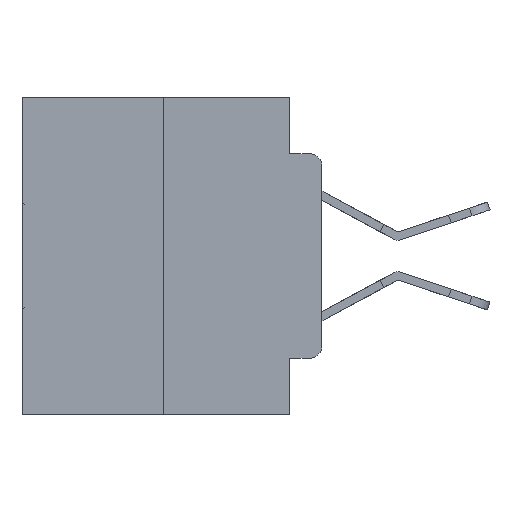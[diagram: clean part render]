
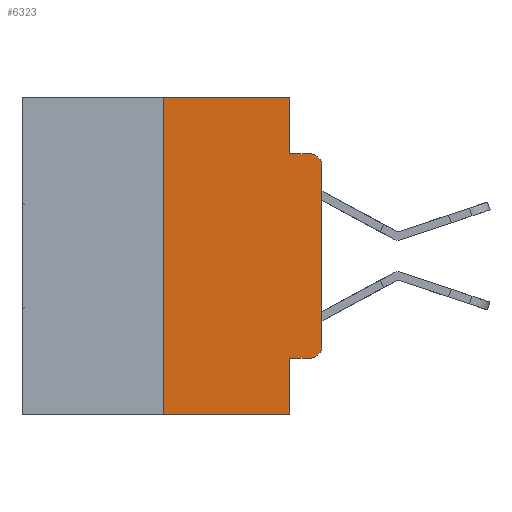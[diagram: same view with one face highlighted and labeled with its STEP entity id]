
A CAD part, left-side view. The second image highlights one B-rep face of the part: STEP entity #6323.
In plain terms, the highlighted planar face has unit normal (-1, 0, 0).
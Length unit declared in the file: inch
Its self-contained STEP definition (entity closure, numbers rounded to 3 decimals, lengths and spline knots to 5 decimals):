
#49 = CARTESIAN_POINT ( 'NONE',  ( 0., 0.02, -0.3915 ) ) ;
#117 = CARTESIAN_POINT ( 'NONE',  ( 0., 0., 0. ) ) ;
#957 = EDGE_CURVE ( 'NONE', #20070, #7459, #7566, .T. ) ;
#1238 = CARTESIAN_POINT ( 'NONE',  ( 0., 0., -0.3915 ) ) ;
#1252 = EDGE_LOOP ( 'NONE', ( #4710, #22778, #15737, #4703, #14623, #15390, #3046, #19075, #13625, #22520 ) ) ;
#1361 = CARTESIAN_POINT ( 'NONE',  ( 0., 0.051, -0.0885 ) ) ;
#1667 = VECTOR ( 'NONE', #22784, 39.37008 ) ;
#1804 = CARTESIAN_POINT ( 'NONE',  ( 0., 0.25, 0. ) ) ;
#1815 = CARTESIAN_POINT ( 'NONE',  ( 0., 0.02, -0.0885 ) ) ;
#1923 = AXIS2_PLACEMENT_3D ( 'NONE', #9170, #6244, #6087 ) ;
#2115 = VERTEX_POINT ( 'NONE', #1361 ) ;
#2383 = EDGE_CURVE ( 'NONE', #4412, #13299, #23079, .T. ) ;
#2407 = LINE ( 'NONE', #117, #4605 ) ;
#3046 = ORIENTED_EDGE ( 'NONE', *, *, #19888, .T. ) ;
#3507 = VECTOR ( 'NONE', #13472, 39.37008 ) ;
#4167 = DIRECTION ( 'NONE',  ( 0., 0., -1. ) ) ;
#4253 = PLANE ( 'NONE',  #1923 ) ;
#4412 = VERTEX_POINT ( 'NONE', #4802 ) ;
#4605 = VECTOR ( 'NONE', #20945, 39.37008 ) ;
#4703 = ORIENTED_EDGE ( 'NONE', *, *, #20330, .F. ) ;
#4710 = ORIENTED_EDGE ( 'NONE', *, *, #10643, .T. ) ;
#4802 = CARTESIAN_POINT ( 'NONE',  ( 0., 0.25, -0.5 ) ) ;
#5349 = CARTESIAN_POINT ( 'NONE',  ( 0., 0.02, -0.4115 ) ) ;
#6087 = DIRECTION ( 'NONE',  ( 0., 0., -1. ) ) ;
#6143 = DIRECTION ( 'NONE',  ( 0., -1., 0. ) ) ;
#6244 = DIRECTION ( 'NONE',  ( 1., 0., 0. ) ) ;
#6323 = ADVANCED_FACE ( 'NONE', ( #13639 ), #4253, .F. ) ;
#6870 = DIRECTION ( 'NONE',  ( 0., -1., 0. ) ) ;
#7145 = CARTESIAN_POINT ( 'NONE',  ( 0., 0.25, 0. ) ) ;
#7459 = VERTEX_POINT ( 'NONE', #5349 ) ;
#7566 = LINE ( 'NONE', #22283, #10491 ) ;
#7925 = CARTESIAN_POINT ( 'NONE',  ( 0., 0.051, -0.5 ) ) ;
#8088 = EDGE_CURVE ( 'NONE', #19661, #25781, #27586, .T. ) ;
#8768 = CARTESIAN_POINT ( 'NONE',  ( 0., 0.473, 0. ) ) ;
#9170 = CARTESIAN_POINT ( 'NONE',  ( 0., 0.473, 0. ) ) ;
#10226 = VECTOR ( 'NONE', #6143, 39.37008 ) ;
#10491 = VECTOR ( 'NONE', #26886, 39.37008 ) ;
#10643 = EDGE_CURVE ( 'NONE', #29318, #19661, #2407, .T. ) ;
#11443 = DIRECTION ( 'NONE',  ( 0., 0., -1. ) ) ;
#11681 = VERTEX_POINT ( 'NONE', #7925 ) ;
#13299 = VERTEX_POINT ( 'NONE', #7145 ) ;
#13325 = CARTESIAN_POINT ( 'NONE',  ( 0., 0.473, -0.5 ) ) ;
#13472 = DIRECTION ( 'NONE',  ( 0., -1., 0. ) ) ;
#13625 = ORIENTED_EDGE ( 'NONE', *, *, #957, .T. ) ;
#13639 = FACE_OUTER_BOUND ( 'NONE', #1252, .T. ) ;
#14623 = ORIENTED_EDGE ( 'NONE', *, *, #16229, .F. ) ;
#14943 = EDGE_CURVE ( 'NONE', #2115, #25781, #25267, .T. ) ;
#15390 = ORIENTED_EDGE ( 'NONE', *, *, #2383, .F. ) ;
#15695 = LINE ( 'NONE', #22579, #24562 ) ;
#15737 = ORIENTED_EDGE ( 'NONE', *, *, #14943, .F. ) ;
#16229 = EDGE_CURVE ( 'NONE', #13299, #21960, #18280, .T. ) ;
#16376 = EDGE_CURVE ( 'NONE', #7459, #29318, #27823, .T. ) ;
#17322 = DIRECTION ( 'NONE',  ( 0., 0., -1. ) ) ;
#17327 = AXIS2_PLACEMENT_3D ( 'NONE', #20641, #22777, #11443 ) ;
#18280 = LINE ( 'NONE', #8768, #10226 ) ;
#19026 = LINE ( 'NONE', #28359, #22349 ) ;
#19075 = ORIENTED_EDGE ( 'NONE', *, *, #26569, .F. ) ;
#19661 = VERTEX_POINT ( 'NONE', #28821 ) ;
#19888 = EDGE_CURVE ( 'NONE', #4412, #11681, #22803, .T. ) ;
#20070 = VERTEX_POINT ( 'NONE', #23552 ) ;
#20330 = EDGE_CURVE ( 'NONE', #21960, #2115, #15695, .T. ) ;
#20641 = CARTESIAN_POINT ( 'NONE',  ( 0., 0.02, -0.1085 ) ) ;
#20945 = DIRECTION ( 'NONE',  ( 0., 0., 1. ) ) ;
#21171 = DIRECTION ( 'NONE',  ( -1., 0., 0. ) ) ;
#21960 = VERTEX_POINT ( 'NONE', #24122 ) ;
#21979 = VECTOR ( 'NONE', #6870, 39.37008 ) ;
#22283 = CARTESIAN_POINT ( 'NONE',  ( 0., 0.051, -0.4115 ) ) ;
#22349 = VECTOR ( 'NONE', #17322, 39.37008 ) ;
#22520 = ORIENTED_EDGE ( 'NONE', *, *, #16376, .T. ) ;
#22579 = CARTESIAN_POINT ( 'NONE',  ( 0., 0.051, 0. ) ) ;
#22777 = DIRECTION ( 'NONE',  ( -1., 0., 0. ) ) ;
#22778 = ORIENTED_EDGE ( 'NONE', *, *, #8088, .T. ) ;
#22784 = DIRECTION ( 'NONE',  ( 0., 0., 1. ) ) ;
#22803 = LINE ( 'NONE', #13325, #3507 ) ;
#23079 = LINE ( 'NONE', #1804, #1667 ) ;
#23552 = CARTESIAN_POINT ( 'NONE',  ( 0., 0.051, -0.4115 ) ) ;
#24122 = CARTESIAN_POINT ( 'NONE',  ( 0., 0.051, 0. ) ) ;
#24562 = VECTOR ( 'NONE', #4167, 39.37008 ) ;
#25267 = LINE ( 'NONE', #25567, #21979 ) ;
#25567 = CARTESIAN_POINT ( 'NONE',  ( 0., 0.051, -0.0885 ) ) ;
#25781 = VERTEX_POINT ( 'NONE', #1815 ) ;
#26569 = EDGE_CURVE ( 'NONE', #20070, #11681, #19026, .T. ) ;
#26886 = DIRECTION ( 'NONE',  ( 0., -1., 0. ) ) ;
#27586 = CIRCLE ( 'NONE', #17327, 0.02 ) ;
#27764 = DIRECTION ( 'NONE',  ( 0., 0., -1. ) ) ;
#27823 = CIRCLE ( 'NONE', #29301, 0.02 ) ;
#28359 = CARTESIAN_POINT ( 'NONE',  ( 0., 0.051, 0. ) ) ;
#28821 = CARTESIAN_POINT ( 'NONE',  ( 0., 0., -0.1085 ) ) ;
#29301 = AXIS2_PLACEMENT_3D ( 'NONE', #49, #21171, #27764 ) ;
#29318 = VERTEX_POINT ( 'NONE', #1238 ) ;
